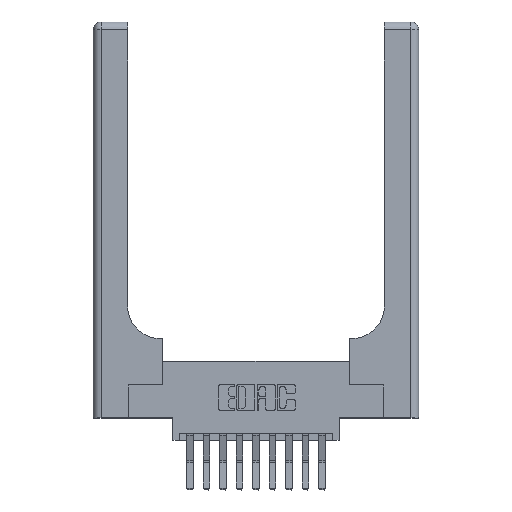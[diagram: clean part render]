
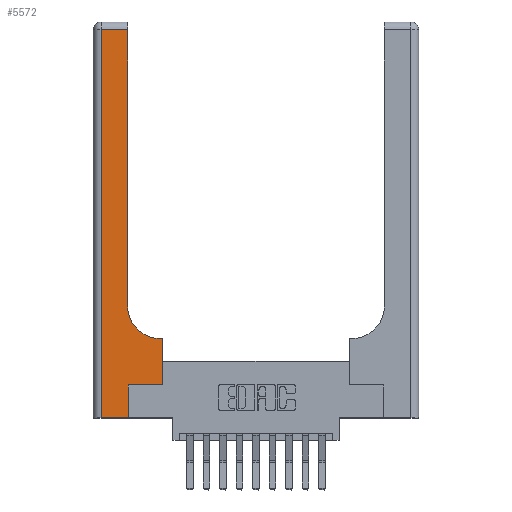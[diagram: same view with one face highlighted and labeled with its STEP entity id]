
A CAD part, top view. The second image highlights one B-rep face of the part: STEP entity #5572.
In plain terms, the highlighted planar face has unit normal (0, 0, 1).
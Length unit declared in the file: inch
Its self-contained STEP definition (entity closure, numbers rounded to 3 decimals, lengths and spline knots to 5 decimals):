
#352 = LINE ( 'NONE', #10244, #12277 ) ;
#902 = CARTESIAN_POINT ( 'NONE',  ( 0.51, 0.85, 0.37 ) ) ;
#1220 = PLANE ( 'NONE',  #6091 ) ;
#1298 = VERTEX_POINT ( 'NONE', #16139 ) ;
#2234 = LINE ( 'NONE', #5919, #9781 ) ;
#2446 = FACE_OUTER_BOUND ( 'NONE', #3162, .T. ) ;
#2620 = VECTOR ( 'NONE', #14720, 39.37008 ) ;
#2758 = DIRECTION ( 'NONE',  ( -1., 0., 0. ) ) ;
#2790 = CARTESIAN_POINT ( 'NONE',  ( 0.265, 0., 0.37 ) ) ;
#3162 = EDGE_LOOP ( 'NONE', ( #4419, #7592, #8503, #8122, #4695, #16145, #5318, #11797, #5180 ) ) ;
#3394 = VERTEX_POINT ( 'NONE', #12663 ) ;
#3575 = VERTEX_POINT ( 'NONE', #10508 ) ;
#3637 = EDGE_CURVE ( 'NONE', #6175, #3575, #15820, .T. ) ;
#3909 = EDGE_CURVE ( 'NONE', #5134, #5260, #11829, .T. ) ;
#4419 = ORIENTED_EDGE ( 'NONE', *, *, #3637, .T. ) ;
#4522 = LINE ( 'NONE', #14633, #2620 ) ;
#4551 = VECTOR ( 'NONE', #8268, 39.37008 ) ;
#4650 = DIRECTION ( 'NONE',  ( 0., 1., 0. ) ) ;
#4695 = ORIENTED_EDGE ( 'NONE', *, *, #11136, .T. ) ;
#4974 = VECTOR ( 'NONE', #5801, 39.37008 ) ;
#4983 = EDGE_CURVE ( 'NONE', #5975, #11833, #9174, .T. ) ;
#5134 = VERTEX_POINT ( 'NONE', #13646 ) ;
#5180 = ORIENTED_EDGE ( 'NONE', *, *, #8307, .T. ) ;
#5260 = VERTEX_POINT ( 'NONE', #8920 ) ;
#5318 = ORIENTED_EDGE ( 'NONE', *, *, #4983, .T. ) ;
#5572 = ADVANCED_FACE ( 'NONE', ( #2446 ), #1220, .F. ) ;
#5711 = CARTESIAN_POINT ( 'NONE',  ( 0.26, 3., 0.37 ) ) ;
#5788 = DIRECTION ( 'NONE',  ( -1., 0., 0. ) ) ;
#5801 = DIRECTION ( 'NONE',  ( 0., 1., 0. ) ) ;
#5919 = CARTESIAN_POINT ( 'NONE',  ( 0., 0., 0.37 ) ) ;
#5975 = VERTEX_POINT ( 'NONE', #9763 ) ;
#6088 = DIRECTION ( 'NONE',  ( 1., 0., 0. ) ) ;
#6091 = AXIS2_PLACEMENT_3D ( 'NONE', #9545, #7358, #6211 ) ;
#6175 = VERTEX_POINT ( 'NONE', #9035 ) ;
#6211 = DIRECTION ( 'NONE',  ( -1., 0., 0. ) ) ;
#7222 = DIRECTION ( 'NONE',  ( 1., 0., 0. ) ) ;
#7358 = DIRECTION ( 'NONE',  ( 0., 0., -1. ) ) ;
#7487 = CIRCLE ( 'NONE', #9538, 0.25 ) ;
#7592 = ORIENTED_EDGE ( 'NONE', *, *, #11700, .T. ) ;
#7725 = VECTOR ( 'NONE', #4650, 39.37008 ) ;
#7859 = EDGE_CURVE ( 'NONE', #5260, #15418, #2234, .T. ) ;
#7959 = CARTESIAN_POINT ( 'NONE',  ( 0.528, 0.25, 0.37 ) ) ;
#8122 = ORIENTED_EDGE ( 'NONE', *, *, #7859, .T. ) ;
#8268 = DIRECTION ( 'NONE',  ( 0., -1., 0. ) ) ;
#8307 = EDGE_CURVE ( 'NONE', #3394, #6175, #7487, .T. ) ;
#8503 = ORIENTED_EDGE ( 'NONE', *, *, #3909, .T. ) ;
#8920 = CARTESIAN_POINT ( 'NONE',  ( 0.06, 0., 0.37 ) ) ;
#9035 = CARTESIAN_POINT ( 'NONE',  ( 0.26, 0.85, 0.37 ) ) ;
#9174 = LINE ( 'NONE', #7959, #11007 ) ;
#9538 = AXIS2_PLACEMENT_3D ( 'NONE', #902, #14798, #7222 ) ;
#9545 = CARTESIAN_POINT ( 'NONE',  ( 0., 3., 0.37 ) ) ;
#9763 = CARTESIAN_POINT ( 'NONE',  ( 0.528, 0.25, 0.37 ) ) ;
#9781 = VECTOR ( 'NONE', #6088, 39.37008 ) ;
#10244 = CARTESIAN_POINT ( 'NONE',  ( 0., 2.94, 0.37 ) ) ;
#10508 = CARTESIAN_POINT ( 'NONE',  ( 0.26, 2.94, 0.37 ) ) ;
#11007 = VECTOR ( 'NONE', #13079, 39.37008 ) ;
#11136 = EDGE_CURVE ( 'NONE', #15418, #1298, #13232, .T. ) ;
#11700 = EDGE_CURVE ( 'NONE', #3575, #5134, #352, .T. ) ;
#11797 = ORIENTED_EDGE ( 'NONE', *, *, #15484, .T. ) ;
#11829 = LINE ( 'NONE', #14300, #4551 ) ;
#11833 = VERTEX_POINT ( 'NONE', #13026 ) ;
#11906 = CARTESIAN_POINT ( 'NONE',  ( 0.265, 0., 0.37 ) ) ;
#12146 = CARTESIAN_POINT ( 'NONE',  ( 0.26, 0.6, 0.37 ) ) ;
#12277 = VECTOR ( 'NONE', #2758, 39.37008 ) ;
#12473 = EDGE_CURVE ( 'NONE', #1298, #5975, #4522, .T. ) ;
#12663 = CARTESIAN_POINT ( 'NONE',  ( 0.51, 0.6, 0.37 ) ) ;
#13026 = CARTESIAN_POINT ( 'NONE',  ( 0.528, 0.6, 0.37 ) ) ;
#13079 = DIRECTION ( 'NONE',  ( 0., 1., 0. ) ) ;
#13099 = VECTOR ( 'NONE', #5788, 39.37008 ) ;
#13232 = LINE ( 'NONE', #11906, #4974 ) ;
#13646 = CARTESIAN_POINT ( 'NONE',  ( 0.06, 2.94, 0.37 ) ) ;
#14300 = CARTESIAN_POINT ( 'NONE',  ( 0.06, 3., 0.37 ) ) ;
#14633 = CARTESIAN_POINT ( 'NONE',  ( 0.265, 0.25, 0.37 ) ) ;
#14720 = DIRECTION ( 'NONE',  ( 1., 0., 0. ) ) ;
#14798 = DIRECTION ( 'NONE',  ( 0., 0., -1. ) ) ;
#15418 = VERTEX_POINT ( 'NONE', #2790 ) ;
#15484 = EDGE_CURVE ( 'NONE', #11833, #3394, #15819, .T. ) ;
#15819 = LINE ( 'NONE', #12146, #13099 ) ;
#15820 = LINE ( 'NONE', #5711, #7725 ) ;
#16139 = CARTESIAN_POINT ( 'NONE',  ( 0.265, 0.25, 0.37 ) ) ;
#16145 = ORIENTED_EDGE ( 'NONE', *, *, #12473, .T. ) ;
